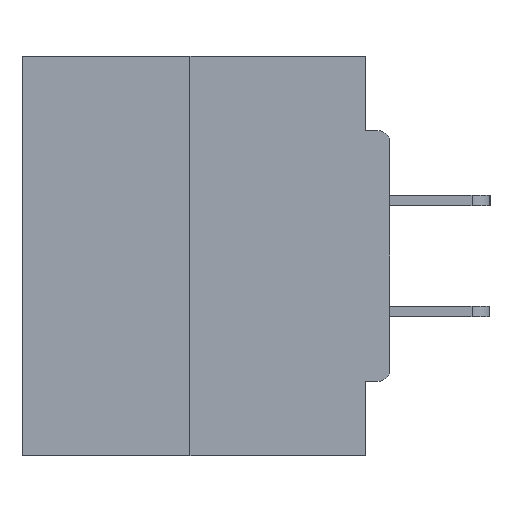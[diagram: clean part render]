
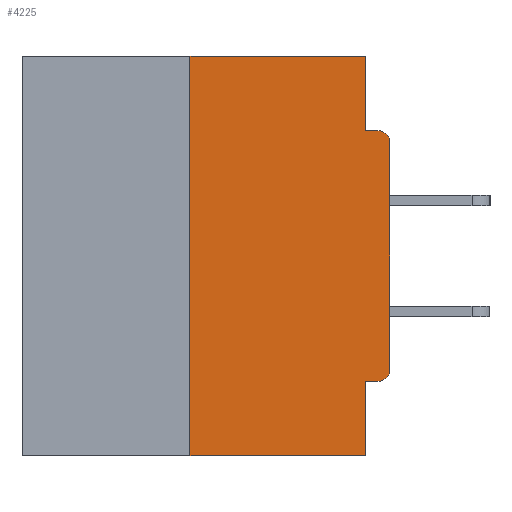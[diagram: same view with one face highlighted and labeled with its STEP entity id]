
A CAD part, left-side view. The second image highlights one B-rep face of the part: STEP entity #4225.
In plain terms, the highlighted planar face has unit normal (-1, 0, 0).
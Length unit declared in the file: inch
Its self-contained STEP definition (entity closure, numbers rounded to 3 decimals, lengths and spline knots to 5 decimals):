
#878 = DIRECTION ( 'NONE',  ( 0., 0., -1. ) ) ;
#977 = AXIS2_PLACEMENT_3D ( 'NONE', #2430, #2198, #17363 ) ;
#1668 = AXIS2_PLACEMENT_3D ( 'NONE', #27339, #32614, #13739 ) ;
#1670 = EDGE_CURVE ( 'NONE', #25444, #31749, #14863, .T. ) ;
#2001 = CARTESIAN_POINT ( 'NONE',  ( 0., 0.015, -0.0935 ) ) ;
#2189 = DIRECTION ( 'NONE',  ( 0., 1., 0. ) ) ;
#2198 = DIRECTION ( 'NONE',  ( 1., 0., 0. ) ) ;
#2430 = CARTESIAN_POINT ( 'NONE',  ( 0., 0.46, 0. ) ) ;
#2580 = EDGE_CURVE ( 'NONE', #20069, #32801, #17790, .T. ) ;
#2852 = ORIENTED_EDGE ( 'NONE', *, *, #23469, .F. ) ;
#3885 = DIRECTION ( 'NONE',  ( -1., 0., 0. ) ) ;
#3939 = VECTOR ( 'NONE', #23919, 39.37008 ) ;
#4225 = ADVANCED_FACE ( 'NONE', ( #9079 ), #32762, .F. ) ;
#4662 = DIRECTION ( 'NONE',  ( 0., 0., -1. ) ) ;
#5074 = CARTESIAN_POINT ( 'NONE',  ( 0., 0.25, 0. ) ) ;
#5323 = VECTOR ( 'NONE', #4662, 39.37008 ) ;
#6429 = EDGE_LOOP ( 'NONE', ( #2852, #23913, #16032, #7671, #7530, #14844, #25093, #15655, #28820, #29302 ) ) ;
#7098 = VERTEX_POINT ( 'NONE', #34614 ) ;
#7530 = ORIENTED_EDGE ( 'NONE', *, *, #31249, .F. ) ;
#7671 = ORIENTED_EDGE ( 'NONE', *, *, #1670, .F. ) ;
#7719 = VERTEX_POINT ( 'NONE', #13675 ) ;
#8030 = VECTOR ( 'NONE', #878, 39.37008 ) ;
#8595 = VECTOR ( 'NONE', #34330, 39.37008 ) ;
#9079 = FACE_OUTER_BOUND ( 'NONE', #6429, .T. ) ;
#9495 = CARTESIAN_POINT ( 'NONE',  ( 0., 0., -0.0935 ) ) ;
#10273 = CARTESIAN_POINT ( 'NONE',  ( 0., 0., -0.1085 ) ) ;
#10348 = VECTOR ( 'NONE', #20512, 39.37008 ) ;
#10954 = EDGE_CURVE ( 'NONE', #7719, #31749, #24858, .T. ) ;
#11078 = EDGE_CURVE ( 'NONE', #7719, #24879, #17611, .T. ) ;
#11995 = CARTESIAN_POINT ( 'NONE',  ( 0., 0., -0.3915 ) ) ;
#12362 = LINE ( 'NONE', #33074, #22212 ) ;
#12576 = LINE ( 'NONE', #29318, #5323 ) ;
#12874 = VERTEX_POINT ( 'NONE', #2001 ) ;
#13094 = VECTOR ( 'NONE', #2189, 39.37008 ) ;
#13351 = LINE ( 'NONE', #9495, #10348 ) ;
#13394 = CIRCLE ( 'NONE', #17248, 0.015 ) ;
#13675 = CARTESIAN_POINT ( 'NONE',  ( 0., 0.25, -0.5 ) ) ;
#13739 = DIRECTION ( 'NONE',  ( 0., 0., -1. ) ) ;
#14844 = ORIENTED_EDGE ( 'NONE', *, *, #20681, .T. ) ;
#14863 = LINE ( 'NONE', #17178, #8030 ) ;
#15655 = ORIENTED_EDGE ( 'NONE', *, *, #15711, .T. ) ;
#15711 = EDGE_CURVE ( 'NONE', #32801, #12874, #20627, .T. ) ;
#15813 = EDGE_CURVE ( 'NONE', #29187, #12874, #13351, .T. ) ;
#16032 = ORIENTED_EDGE ( 'NONE', *, *, #10954, .T. ) ;
#17178 = CARTESIAN_POINT ( 'NONE',  ( 0., 0.031, -0.5 ) ) ;
#17248 = AXIS2_PLACEMENT_3D ( 'NONE', #34175, #3885, #22977 ) ;
#17363 = DIRECTION ( 'NONE',  ( 0., 0., -1. ) ) ;
#17611 = LINE ( 'NONE', #5074, #3939 ) ;
#17790 = LINE ( 'NONE', #25630, #30157 ) ;
#17828 = CARTESIAN_POINT ( 'NONE',  ( 0., 0.46, -0.5 ) ) ;
#18495 = CARTESIAN_POINT ( 'NONE',  ( 0., 0., -0.4065 ) ) ;
#18611 = CARTESIAN_POINT ( 'NONE',  ( 0., 0.031, -0.4065 ) ) ;
#19653 = CARTESIAN_POINT ( 'NONE',  ( 0., 0.031, -0.0935 ) ) ;
#20069 = VERTEX_POINT ( 'NONE', #11995 ) ;
#20389 = DIRECTION ( 'NONE',  ( 0., 0., 1. ) ) ;
#20512 = DIRECTION ( 'NONE',  ( 0., -1., 0. ) ) ;
#20627 = CIRCLE ( 'NONE', #1668, 0.015 ) ;
#20681 = EDGE_CURVE ( 'NONE', #20904, #20069, #13394, .T. ) ;
#20904 = VERTEX_POINT ( 'NONE', #21397 ) ;
#21397 = CARTESIAN_POINT ( 'NONE',  ( 0., 0.015, -0.4065 ) ) ;
#22212 = VECTOR ( 'NONE', #27801, 39.37008 ) ;
#22977 = DIRECTION ( 'NONE',  ( 0., 0., -1. ) ) ;
#23469 = EDGE_CURVE ( 'NONE', #24879, #7098, #12362, .T. ) ;
#23913 = ORIENTED_EDGE ( 'NONE', *, *, #11078, .F. ) ;
#23919 = DIRECTION ( 'NONE',  ( 0., 0., 1. ) ) ;
#24858 = LINE ( 'NONE', #17828, #8595 ) ;
#24879 = VERTEX_POINT ( 'NONE', #34989 ) ;
#25093 = ORIENTED_EDGE ( 'NONE', *, *, #2580, .T. ) ;
#25444 = VERTEX_POINT ( 'NONE', #18611 ) ;
#25630 = CARTESIAN_POINT ( 'NONE',  ( 0., 0., 0. ) ) ;
#25812 = CARTESIAN_POINT ( 'NONE',  ( 0., 0.031, -0.5 ) ) ;
#27157 = LINE ( 'NONE', #18495, #13094 ) ;
#27339 = CARTESIAN_POINT ( 'NONE',  ( 0., 0.015, -0.1085 ) ) ;
#27801 = DIRECTION ( 'NONE',  ( 0., -1., 0. ) ) ;
#28820 = ORIENTED_EDGE ( 'NONE', *, *, #15813, .F. ) ;
#29187 = VERTEX_POINT ( 'NONE', #19653 ) ;
#29302 = ORIENTED_EDGE ( 'NONE', *, *, #32466, .F. ) ;
#29318 = CARTESIAN_POINT ( 'NONE',  ( 0., 0.031, 0. ) ) ;
#30157 = VECTOR ( 'NONE', #20389, 39.37008 ) ;
#31249 = EDGE_CURVE ( 'NONE', #20904, #25444, #27157, .T. ) ;
#31749 = VERTEX_POINT ( 'NONE', #25812 ) ;
#32466 = EDGE_CURVE ( 'NONE', #7098, #29187, #12576, .T. ) ;
#32614 = DIRECTION ( 'NONE',  ( -1., 0., 0. ) ) ;
#32762 = PLANE ( 'NONE',  #977 ) ;
#32801 = VERTEX_POINT ( 'NONE', #10273 ) ;
#33074 = CARTESIAN_POINT ( 'NONE',  ( 0., 0.46, 0. ) ) ;
#34175 = CARTESIAN_POINT ( 'NONE',  ( 0., 0.015, -0.3915 ) ) ;
#34330 = DIRECTION ( 'NONE',  ( 0., -1., 0. ) ) ;
#34614 = CARTESIAN_POINT ( 'NONE',  ( 0., 0.031, 0. ) ) ;
#34989 = CARTESIAN_POINT ( 'NONE',  ( 0., 0.25, 0. ) ) ;
